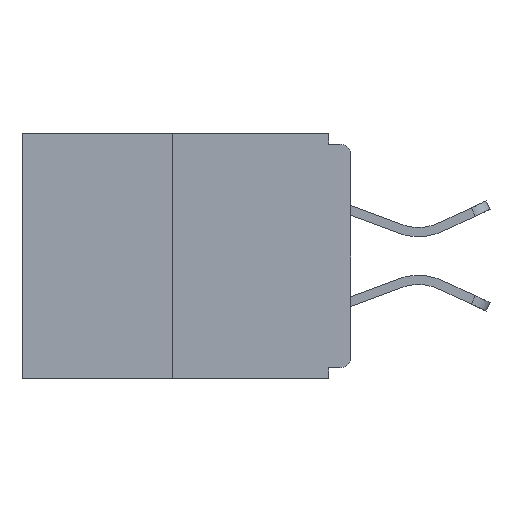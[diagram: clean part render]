
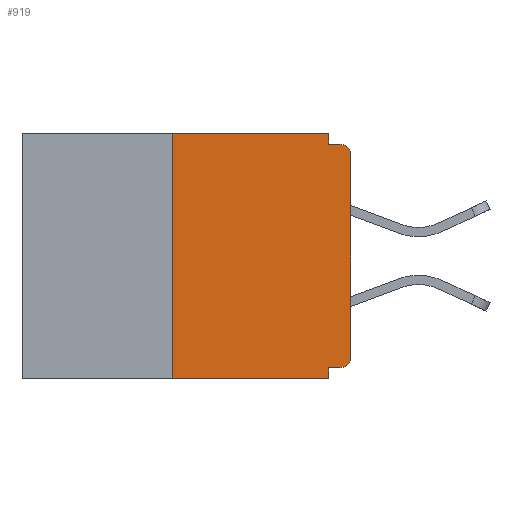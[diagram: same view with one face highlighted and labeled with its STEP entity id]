
A CAD part, left-side view. The second image highlights one B-rep face of the part: STEP entity #919.
In plain terms, the highlighted planar face has unit normal (-1, 0, 0).
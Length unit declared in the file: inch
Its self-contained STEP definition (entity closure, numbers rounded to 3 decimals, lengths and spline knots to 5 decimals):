
#308 = CARTESIAN_POINT ( 'NONE',  ( 0., 0.015, -0.015 ) ) ;
#343 = CARTESIAN_POINT ( 'NONE',  ( 0., 0.015, -0.328 ) ) ;
#919 = ADVANCED_FACE ( 'NONE', ( #12520 ), #12531, .F. ) ;
#1056 = VERTEX_POINT ( 'NONE', #7597 ) ;
#1178 = AXIS2_PLACEMENT_3D ( 'NONE', #7187, #10390, #10473 ) ;
#1275 = CARTESIAN_POINT ( 'NONE',  ( 0., 0.25, -0.343 ) ) ;
#1323 = ORIENTED_EDGE ( 'NONE', *, *, #5522, .F. ) ;
#1490 = CARTESIAN_POINT ( 'NONE',  ( 0., 0., 0. ) ) ;
#1698 = VERTEX_POINT ( 'NONE', #3023 ) ;
#1744 = LINE ( 'NONE', #10111, #12849 ) ;
#1890 = DIRECTION ( 'NONE',  ( 0., 0., 1. ) ) ;
#2098 = EDGE_CURVE ( 'NONE', #6488, #4848, #6428, .T. ) ;
#2147 = CARTESIAN_POINT ( 'NONE',  ( 0., 0., -0.328 ) ) ;
#2190 = LINE ( 'NONE', #9165, #7741 ) ;
#2311 = VERTEX_POINT ( 'NONE', #308 ) ;
#2491 = DIRECTION ( 'NONE',  ( 0., 0., -1. ) ) ;
#2511 = CARTESIAN_POINT ( 'NONE',  ( 0., 0.031, -0.015 ) ) ;
#2802 = ORIENTED_EDGE ( 'NONE', *, *, #5080, .F. ) ;
#2819 = LINE ( 'NONE', #1490, #8184 ) ;
#2941 = EDGE_CURVE ( 'NONE', #13527, #2311, #2190, .T. ) ;
#3023 = CARTESIAN_POINT ( 'NONE',  ( 0., 0., -0.03 ) ) ;
#3119 = ORIENTED_EDGE ( 'NONE', *, *, #2098, .F. ) ;
#3335 = CARTESIAN_POINT ( 'NONE',  ( 0., 0.031, 0. ) ) ;
#3627 = CARTESIAN_POINT ( 'NONE',  ( 0., 0.015, -0.313 ) ) ;
#3671 = CARTESIAN_POINT ( 'NONE',  ( 0., 0.015, -0.03 ) ) ;
#3730 = ORIENTED_EDGE ( 'NONE', *, *, #6002, .T. ) ;
#3874 = CARTESIAN_POINT ( 'NONE',  ( 0., 0.25, 0. ) ) ;
#3924 = VECTOR ( 'NONE', #8754, 39.37008 ) ;
#3939 = DIRECTION ( 'NONE',  ( 0., -1., 0. ) ) ;
#4108 = EDGE_CURVE ( 'NONE', #4252, #7719, #8787, .T. ) ;
#4154 = EDGE_CURVE ( 'NONE', #1698, #2311, #10918, .T. ) ;
#4252 = VERTEX_POINT ( 'NONE', #343 ) ;
#4284 = VECTOR ( 'NONE', #13434, 39.37008 ) ;
#4848 = VERTEX_POINT ( 'NONE', #7132 ) ;
#5080 = EDGE_CURVE ( 'NONE', #5540, #13527, #12533, .T. ) ;
#5522 = EDGE_CURVE ( 'NONE', #4252, #6488, #6642, .T. ) ;
#5540 = VERTEX_POINT ( 'NONE', #3335 ) ;
#5761 = EDGE_CURVE ( 'NONE', #1056, #5540, #1744, .T. ) ;
#5914 = ORIENTED_EDGE ( 'NONE', *, *, #4154, .T. ) ;
#6002 = EDGE_CURVE ( 'NONE', #8694, #4848, #13183, .T. ) ;
#6428 = LINE ( 'NONE', #12366, #12815 ) ;
#6488 = VERTEX_POINT ( 'NONE', #9604 ) ;
#6642 = LINE ( 'NONE', #2147, #3924 ) ;
#6853 = DIRECTION ( 'NONE',  ( 0., 0., 1. ) ) ;
#6973 = ORIENTED_EDGE ( 'NONE', *, *, #10320, .F. ) ;
#7132 = CARTESIAN_POINT ( 'NONE',  ( 0., 0.031, -0.343 ) ) ;
#7187 = CARTESIAN_POINT ( 'NONE',  ( 0., 0.46, 0. ) ) ;
#7235 = ORIENTED_EDGE ( 'NONE', *, *, #5761, .F. ) ;
#7597 = CARTESIAN_POINT ( 'NONE',  ( 0., 0.25, 0. ) ) ;
#7719 = VERTEX_POINT ( 'NONE', #8348 ) ;
#7741 = VECTOR ( 'NONE', #11257, 39.37008 ) ;
#7846 = DIRECTION ( 'NONE',  ( -1., 0., 0. ) ) ;
#8087 = DIRECTION ( 'NONE',  ( 0., -1., 0. ) ) ;
#8184 = VECTOR ( 'NONE', #6853, 39.37008 ) ;
#8348 = CARTESIAN_POINT ( 'NONE',  ( 0., 0., -0.313 ) ) ;
#8694 = VERTEX_POINT ( 'NONE', #1275 ) ;
#8754 = DIRECTION ( 'NONE',  ( 0., 1., 0. ) ) ;
#8787 = CIRCLE ( 'NONE', #13975, 0.015 ) ;
#9165 = CARTESIAN_POINT ( 'NONE',  ( 0., 0., -0.015 ) ) ;
#9253 = ORIENTED_EDGE ( 'NONE', *, *, #2941, .F. ) ;
#9363 = AXIS2_PLACEMENT_3D ( 'NONE', #3671, #11203, #2491 ) ;
#9593 = LINE ( 'NONE', #3874, #11588 ) ;
#9604 = CARTESIAN_POINT ( 'NONE',  ( 0., 0.031, -0.328 ) ) ;
#9932 = ORIENTED_EDGE ( 'NONE', *, *, #4108, .T. ) ;
#10111 = CARTESIAN_POINT ( 'NONE',  ( 0., 0.46, 0. ) ) ;
#10226 = CARTESIAN_POINT ( 'NONE',  ( 0., 0.031, 0. ) ) ;
#10267 = DIRECTION ( 'NONE',  ( 0., 0., -1. ) ) ;
#10320 = EDGE_CURVE ( 'NONE', #8694, #1056, #9593, .T. ) ;
#10390 = DIRECTION ( 'NONE',  ( 1., 0., 0. ) ) ;
#10409 = CARTESIAN_POINT ( 'NONE',  ( 0., 0.46, -0.343 ) ) ;
#10453 = EDGE_LOOP ( 'NONE', ( #7235, #6973, #3730, #3119, #1323, #9932, #10492, #5914, #9253, #2802 ) ) ;
#10473 = DIRECTION ( 'NONE',  ( 0., 0., -1. ) ) ;
#10492 = ORIENTED_EDGE ( 'NONE', *, *, #11952, .T. ) ;
#10918 = CIRCLE ( 'NONE', #9363, 0.015 ) ;
#11203 = DIRECTION ( 'NONE',  ( -1., 0., 0. ) ) ;
#11257 = DIRECTION ( 'NONE',  ( 0., -1., 0. ) ) ;
#11503 = VECTOR ( 'NONE', #3939, 39.37008 ) ;
#11588 = VECTOR ( 'NONE', #1890, 39.37008 ) ;
#11952 = EDGE_CURVE ( 'NONE', #7719, #1698, #2819, .T. ) ;
#12366 = CARTESIAN_POINT ( 'NONE',  ( 0., 0.031, -0.343 ) ) ;
#12520 = FACE_OUTER_BOUND ( 'NONE', #10453, .T. ) ;
#12531 = PLANE ( 'NONE',  #1178 ) ;
#12533 = LINE ( 'NONE', #10226, #4284 ) ;
#12815 = VECTOR ( 'NONE', #10267, 39.37008 ) ;
#12849 = VECTOR ( 'NONE', #8087, 39.37008 ) ;
#13183 = LINE ( 'NONE', #10409, #11503 ) ;
#13275 = DIRECTION ( 'NONE',  ( 0., 0., -1. ) ) ;
#13434 = DIRECTION ( 'NONE',  ( 0., 0., -1. ) ) ;
#13527 = VERTEX_POINT ( 'NONE', #2511 ) ;
#13975 = AXIS2_PLACEMENT_3D ( 'NONE', #3627, #7846, #13275 ) ;
